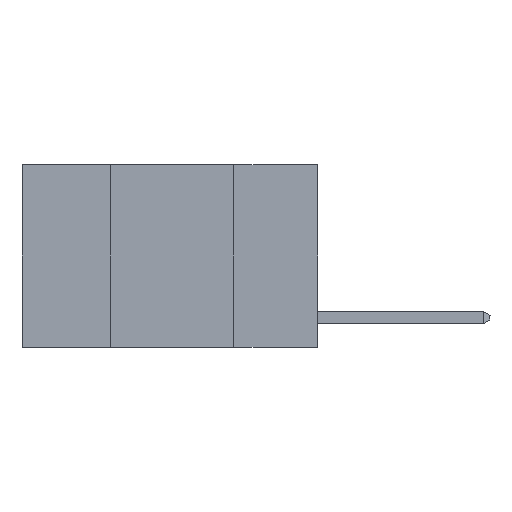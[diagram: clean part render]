
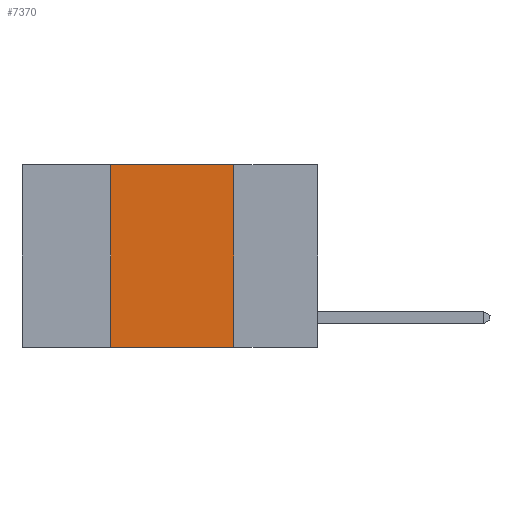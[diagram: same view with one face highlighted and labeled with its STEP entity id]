
A CAD part, left-side view. The second image highlights one B-rep face of the part: STEP entity #7370.
In plain terms, the highlighted planar face has unit normal (-1, 0, 0).
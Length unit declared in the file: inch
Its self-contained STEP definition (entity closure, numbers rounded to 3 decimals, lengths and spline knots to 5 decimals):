
#690 = CARTESIAN_POINT ( 'NONE',  ( 0., 0.17, 0. ) ) ;
#1263 = ORIENTED_EDGE ( 'NONE', *, *, #24689, .F. ) ;
#2406 = CARTESIAN_POINT ( 'NONE',  ( 0., 0.6, -0.37 ) ) ;
#2913 = VECTOR ( 'NONE', #20360, 39.37008 ) ;
#2970 = VECTOR ( 'NONE', #24561, 39.37008 ) ;
#4910 = EDGE_CURVE ( 'NONE', #25205, #18346, #15196, .T. ) ;
#5842 = ORIENTED_EDGE ( 'NONE', *, *, #4910, .T. ) ;
#6361 = DIRECTION ( 'NONE',  ( 1., 0., 0. ) ) ;
#7370 = ADVANCED_FACE ( 'NONE', ( #14708 ), #21241, .F. ) ;
#7386 = VECTOR ( 'NONE', #24812, 39.37008 ) ;
#7821 = LINE ( 'NONE', #16296, #2913 ) ;
#7851 = CARTESIAN_POINT ( 'NONE',  ( 0., 0.42, -0.37 ) ) ;
#9750 = EDGE_CURVE ( 'NONE', #25205, #20000, #7821, .T. ) ;
#10137 = CARTESIAN_POINT ( 'NONE',  ( 0., 0.17, 0. ) ) ;
#10425 = ORIENTED_EDGE ( 'NONE', *, *, #9750, .F. ) ;
#11250 = EDGE_CURVE ( 'NONE', #20000, #21112, #14535, .T. ) ;
#11780 = EDGE_LOOP ( 'NONE', ( #1263, #13901, #10425, #5842 ) ) ;
#13901 = ORIENTED_EDGE ( 'NONE', *, *, #11250, .F. ) ;
#14535 = LINE ( 'NONE', #24951, #7386 ) ;
#14571 = CARTESIAN_POINT ( 'NONE',  ( 0., 0.6, 0. ) ) ;
#14708 = FACE_OUTER_BOUND ( 'NONE', #11780, .T. ) ;
#14914 = DIRECTION ( 'NONE',  ( 0., -1., 0. ) ) ;
#15196 = LINE ( 'NONE', #2406, #23887 ) ;
#15700 = CARTESIAN_POINT ( 'NONE',  ( 0., 0.17, -0.37 ) ) ;
#16296 = CARTESIAN_POINT ( 'NONE',  ( 0., 0.42, 0. ) ) ;
#16913 = DIRECTION ( 'NONE',  ( 0., 0., -1. ) ) ;
#18346 = VERTEX_POINT ( 'NONE', #15700 ) ;
#18613 = LINE ( 'NONE', #10137, #2970 ) ;
#20000 = VERTEX_POINT ( 'NONE', #24981 ) ;
#20360 = DIRECTION ( 'NONE',  ( 0., 0., 1. ) ) ;
#21112 = VERTEX_POINT ( 'NONE', #690 ) ;
#21241 = PLANE ( 'NONE',  #21326 ) ;
#21326 = AXIS2_PLACEMENT_3D ( 'NONE', #14571, #6361, #16913 ) ;
#23887 = VECTOR ( 'NONE', #14914, 39.37008 ) ;
#24561 = DIRECTION ( 'NONE',  ( 0., 0., -1. ) ) ;
#24689 = EDGE_CURVE ( 'NONE', #21112, #18346, #18613, .T. ) ;
#24812 = DIRECTION ( 'NONE',  ( 0., -1., 0. ) ) ;
#24951 = CARTESIAN_POINT ( 'NONE',  ( 0., 0.6, 0. ) ) ;
#24981 = CARTESIAN_POINT ( 'NONE',  ( 0., 0.42, 0. ) ) ;
#25205 = VERTEX_POINT ( 'NONE', #7851 ) ;
